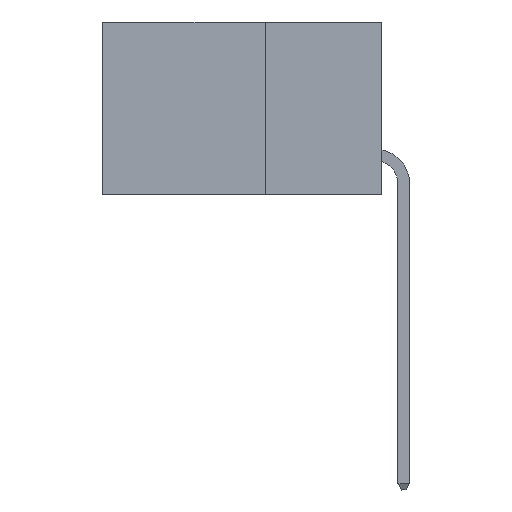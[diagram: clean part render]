
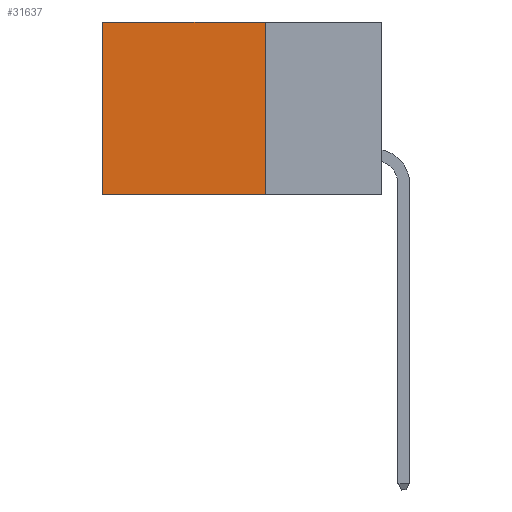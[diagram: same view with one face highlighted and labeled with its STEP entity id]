
A CAD part, left-side view. The second image highlights one B-rep face of the part: STEP entity #31637.
In plain terms, the highlighted planar face has unit normal (-1, 0, 0).
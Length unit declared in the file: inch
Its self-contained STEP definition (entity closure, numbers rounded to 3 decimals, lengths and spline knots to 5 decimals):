
#874 = LINE ( 'NONE', #10695, #32865 ) ;
#1704 = EDGE_LOOP ( 'NONE', ( #34885, #4748, #31775, #27358 ) ) ;
#3480 = DIRECTION ( 'NONE',  ( 1., 0., 0. ) ) ;
#4748 = ORIENTED_EDGE ( 'NONE', *, *, #33437, .F. ) ;
#7505 = DIRECTION ( 'NONE',  ( 0., 0., -1. ) ) ;
#8738 = AXIS2_PLACEMENT_3D ( 'NONE', #23402, #3480, #20202 ) ;
#9777 = DIRECTION ( 'NONE',  ( 0., 0., -1. ) ) ;
#10618 = LINE ( 'NONE', #38162, #33892 ) ;
#10695 = CARTESIAN_POINT ( 'NONE',  ( 0.2875, 0.25, 0. ) ) ;
#10877 = LINE ( 'NONE', #19294, #30003 ) ;
#13005 = VERTEX_POINT ( 'NONE', #30681 ) ;
#13551 = PLANE ( 'NONE',  #8738 ) ;
#15068 = VERTEX_POINT ( 'NONE', #18240 ) ;
#15578 = LINE ( 'NONE', #29561, #24370 ) ;
#15584 = EDGE_CURVE ( 'NONE', #15068, #18058, #874, .T. ) ;
#16888 = CARTESIAN_POINT ( 'NONE',  ( 0.2875, 0.25, -0.37 ) ) ;
#18058 = VERTEX_POINT ( 'NONE', #16888 ) ;
#18240 = CARTESIAN_POINT ( 'NONE',  ( 0.2875, 0.25, 0. ) ) ;
#19294 = CARTESIAN_POINT ( 'NONE',  ( 0.2875, 0.25, -0.37 ) ) ;
#20202 = DIRECTION ( 'NONE',  ( 0., 0., -1. ) ) ;
#20811 = VERTEX_POINT ( 'NONE', #25554 ) ;
#22188 = DIRECTION ( 'NONE',  ( 0., 1., 0. ) ) ;
#23146 = FACE_OUTER_BOUND ( 'NONE', #1704, .T. ) ;
#23402 = CARTESIAN_POINT ( 'NONE',  ( 0.2875, 0.25, 0. ) ) ;
#24370 = VECTOR ( 'NONE', #9777, 39.37008 ) ;
#25323 = EDGE_CURVE ( 'NONE', #15068, #20811, #10618, .T. ) ;
#25554 = CARTESIAN_POINT ( 'NONE',  ( 0.2875, 0.6, 0. ) ) ;
#26511 = DIRECTION ( 'NONE',  ( 0., 1., 0. ) ) ;
#27358 = ORIENTED_EDGE ( 'NONE', *, *, #25323, .T. ) ;
#29561 = CARTESIAN_POINT ( 'NONE',  ( 0.2875, 0.6, 0. ) ) ;
#30003 = VECTOR ( 'NONE', #26511, 39.37008 ) ;
#30681 = CARTESIAN_POINT ( 'NONE',  ( 0.2875, 0.6, -0.37 ) ) ;
#31637 = ADVANCED_FACE ( 'NONE', ( #23146 ), #13551, .F. ) ;
#31775 = ORIENTED_EDGE ( 'NONE', *, *, #15584, .F. ) ;
#32865 = VECTOR ( 'NONE', #7505, 39.37008 ) ;
#33437 = EDGE_CURVE ( 'NONE', #18058, #13005, #10877, .T. ) ;
#33892 = VECTOR ( 'NONE', #22188, 39.37008 ) ;
#34885 = ORIENTED_EDGE ( 'NONE', *, *, #41616, .T. ) ;
#38162 = CARTESIAN_POINT ( 'NONE',  ( 0.2875, 0.25, 0. ) ) ;
#41616 = EDGE_CURVE ( 'NONE', #20811, #13005, #15578, .T. ) ;
